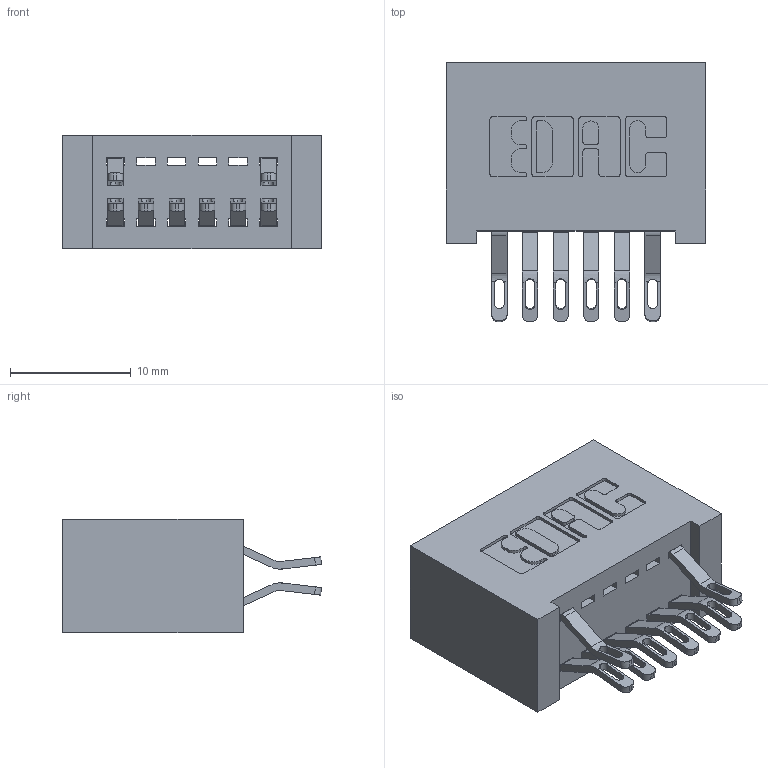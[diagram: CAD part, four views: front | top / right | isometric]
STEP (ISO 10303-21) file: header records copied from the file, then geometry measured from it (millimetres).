
FILE_DESCRIPTION (( 'STEP AP203' ), '1' );
FILE_NAME ('342-012-555-201.STEP', '2018-08-10T15:41:03', ( '' ), ( '' ), 'SwSTEP 2.0', 'SolidWorks 2016', '' );
FILE_SCHEMA (( 'CONFIG_CONTROL_DESIGN' ));
Length unit declared in the file: inch
Products named in the file (3): 342-012-555-201; 342 Part_Lugless; 345-292-001_555 Tail
Assembly tree (9 placements, depth 2):
  342-012-555-201
    342 Part_Lugless
    345-292-001_555 Tail  x8
Bounding box: 21.49 x 21.47 x 9.4 mm (x, y, z)
Volume: 2186.1 mm3; surface area: 2996 mm2
Topology: 9 solids, 9 shells, 590 faces, 1823 edges, 1214 vertices
Faces by surface type: plane 358, cylinder 232
Entity records: 8305 total; most frequent: CARTESIAN_POINT 1468, ORIENTED_EDGE 1378, DIRECTION 1277, EDGE_CURVE 689, LINE 549, VECTOR 549, VERTEX_POINT 458, AXIS2_PLACEMENT_3D 364
